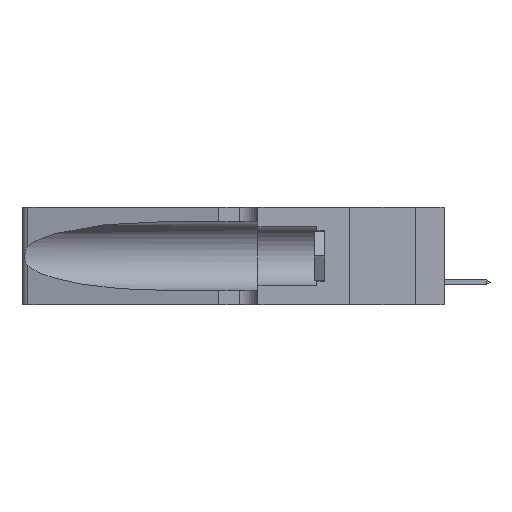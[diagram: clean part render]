
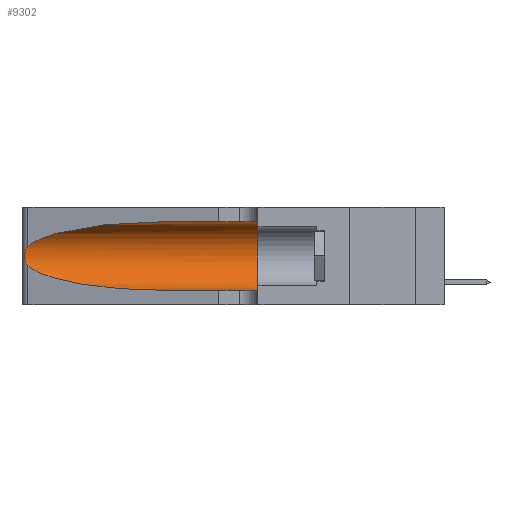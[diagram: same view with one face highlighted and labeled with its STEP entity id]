
A CAD part, left-side view. The second image highlights one B-rep face of the part: STEP entity #9302.
In plain terms, the highlighted cylindrical face has radius 3.308 mm (diameter 6.617 mm), a partial arc.
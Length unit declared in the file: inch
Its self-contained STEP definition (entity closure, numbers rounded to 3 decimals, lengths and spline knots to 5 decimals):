
#2052 = CARTESIAN_POINT ( 'NONE',  ( 0.26075, 1.23896, 0.19203 ) ) ;
#2098 = CARTESIAN_POINT ( 'NONE',  ( 0.2373, 1.15595, 0.08982 ) ) ;
#3570 = CARTESIAN_POINT ( 'NONE',  ( 0.25487, 1.22718, 0.14631 ) ) ;
#4041 = CARTESIAN_POINT ( 'NONE',  ( 0.1305, 0.35, 0.185 ) ) ;
#4953 = CARTESIAN_POINT ( 'NONE',  ( 0.26017, 1.23833, 0.17102 ) ) ;
#5603 = VERTEX_POINT ( 'NONE', #26586 ) ;
#6183 = VERTEX_POINT ( 'NONE', #3570 ) ;
#6469 = CARTESIAN_POINT ( 'NONE',  ( 0.1305, 0.35, 0.31525 ) ) ;
#6683 = VERTEX_POINT ( 'NONE', #33255 ) ;
#7606 = EDGE_CURVE ( 'NONE', #20754, #26557, #24530, .T. ) ;
#7686 = CARTESIAN_POINT ( 'NONE',  ( 0.18966, 0.96281, 0.05475 ) ) ;
#7894 = CARTESIAN_POINT ( 'NONE',  ( 0.25639, 1.23184, 0.21858 ) ) ;
#8058 = CARTESIAN_POINT ( 'NONE',  ( 0.25487, 1.22718, 0.14631 ) ) ;
#9302 = ADVANCED_FACE ( 'NONE', ( #12553 ), #36191, .F. ) ;
#10468 = CARTESIAN_POINT ( 'NONE',  ( 0.25787, 1.23484, 0.2124 ) ) ;
#10715 = CARTESIAN_POINT ( 'NONE',  ( 0.25854, 1.2359, 0.20912 ) ) ;
#10852 = CARTESIAN_POINT ( 'NONE',  ( 0.25856, 1.23593, 0.16098 ) ) ;
#10862 = AXIS2_PLACEMENT_3D ( 'NONE', #4041, #15674, #12991 ) ;
#11027 = CARTESIAN_POINT ( 'NONE',  ( 0.1305, 0.72297, 0.05475 ) ) ;
#11537 = B_SPLINE_CURVE_WITH_KNOTS ( 'NONE', 3,
 ( #13523, #28240, #7894, #10468, #10715, #31073, #2052, #22396, #4953, #10852, #16465, #13778, #33866, #22278 ),
 .UNSPECIFIED., .F., .F.,
 ( 4, 2, 2, 2, 2, 2, 4 ),
 ( 0., 0.00027, 0.00053, 0.00107, 0.0016, 0.00187, 0.00214 ),
 .UNSPECIFIED. ) ;
#11784 = CARTESIAN_POINT ( 'NONE',  ( 0.25487, 1.22718, 0.22369 ) ) ;
#12470 = VECTOR ( 'NONE', #30517, 39.37008 ) ;
#12553 = FACE_OUTER_BOUND ( 'NONE', #32951, .T. ) ;
#12991 = DIRECTION ( 'NONE',  ( 0., 0., 1. ) ) ;
#13214 = CARTESIAN_POINT ( 'NONE',  ( 0.1305, 0.72297, 0.31525 ) ) ;
#13523 = CARTESIAN_POINT ( 'NONE',  ( 0.25487, 1.22718, 0.22369 ) ) ;
#13662 = CARTESIAN_POINT ( 'NONE',  ( 0.1305, 1.61858, 0.185 ) ) ;
#13778 = CARTESIAN_POINT ( 'NONE',  ( 0.25639, 1.23186, 0.15144 ) ) ;
#13784 = VECTOR ( 'NONE', #30299, 39.37008 ) ;
#15674 = DIRECTION ( 'NONE',  ( 0., 1., 0. ) ) ;
#16164 = EDGE_CURVE ( 'NONE', #26557, #6183, #11537, .T. ) ;
#16174 = AXIS2_PLACEMENT_3D ( 'NONE', #13662, #37060, #19612 ) ;
#16465 = CARTESIAN_POINT ( 'NONE',  ( 0.25789, 1.23486, 0.15765 ) ) ;
#16741 = ORIENTED_EDGE ( 'NONE', *, *, #19785, .F. ) ;
#17801 =( BOUNDED_CURVE ( )  B_SPLINE_CURVE ( 3, ( #8058, #2098, #7686, #11027 ),
 .UNSPECIFIED., .F., .F. ) 
 B_SPLINE_CURVE_WITH_KNOTS ( ( 4, 4 ),
 ( 3.44316, 4.71239 ),
 .UNSPECIFIED. ) 
 CURVE ( )  GEOMETRIC_REPRESENTATION_ITEM ( )  RATIONAL_B_SPLINE_CURVE ( ( 1., 0.87, 0.87, 1. ) ) 
 REPRESENTATION_ITEM ( '' )  );
#18469 = CARTESIAN_POINT ( 'NONE',  ( 0.18966, 0.96281, 0.31525 ) ) ;
#18583 = CARTESIAN_POINT ( 'NONE',  ( 0.2373, 1.15595, 0.28018 ) ) ;
#18840 = CARTESIAN_POINT ( 'NONE',  ( 0.25487, 1.22718, 0.22369 ) ) ;
#19612 = DIRECTION ( 'NONE',  ( 0., 0., -1. ) ) ;
#19785 = EDGE_CURVE ( 'NONE', #20754, #27251, #35129, .T. ) ;
#20754 = VERTEX_POINT ( 'NONE', #13214 ) ;
#22278 = CARTESIAN_POINT ( 'NONE',  ( 0.25487, 1.22718, 0.14631 ) ) ;
#22396 = CARTESIAN_POINT ( 'NONE',  ( 0.26075, 1.23896, 0.178 ) ) ;
#22849 = EDGE_CURVE ( 'NONE', #6183, #6683, #17801, .T. ) ;
#23827 = EDGE_CURVE ( 'NONE', #6683, #5603, #36107, .T. ) ;
#24530 =( BOUNDED_CURVE ( )  B_SPLINE_CURVE ( 3, ( #27475, #18469, #18583, #18840 ),
 .UNSPECIFIED., .F., .F. ) 
 B_SPLINE_CURVE_WITH_KNOTS ( ( 4, 4 ),
 ( 1.5708, 2.84003 ),
 .UNSPECIFIED. ) 
 CURVE ( )  GEOMETRIC_REPRESENTATION_ITEM ( )  RATIONAL_B_SPLINE_CURVE ( ( 1., 0.87, 0.87, 1. ) ) 
 REPRESENTATION_ITEM ( '' )  );
#26557 = VERTEX_POINT ( 'NONE', #11784 ) ;
#26586 = CARTESIAN_POINT ( 'NONE',  ( 0.1305, 0.35, 0.05475 ) ) ;
#27251 = VERTEX_POINT ( 'NONE', #6469 ) ;
#27475 = CARTESIAN_POINT ( 'NONE',  ( 0.1305, 0.72297, 0.31525 ) ) ;
#28240 = CARTESIAN_POINT ( 'NONE',  ( 0.25555, 1.22994, 0.2215 ) ) ;
#28391 = ORIENTED_EDGE ( 'NONE', *, *, #22849, .T. ) ;
#28420 = ORIENTED_EDGE ( 'NONE', *, *, #16164, .T. ) ;
#30299 = DIRECTION ( 'NONE',  ( 0., -1., 0. ) ) ;
#30517 = DIRECTION ( 'NONE',  ( 0., -1., 0. ) ) ;
#31073 = CARTESIAN_POINT ( 'NONE',  ( 0.26018, 1.23835, 0.19895 ) ) ;
#32101 = EDGE_CURVE ( 'NONE', #27251, #5603, #33586, .T. ) ;
#32935 = CARTESIAN_POINT ( 'NONE',  ( 0.1305, 1.61858, 0.05475 ) ) ;
#32951 = EDGE_LOOP ( 'NONE', ( #35219, #28420, #28391, #34646, #33356, #16741 ) ) ;
#33096 = CARTESIAN_POINT ( 'NONE',  ( 0.1305, 1.61858, 0.31525 ) ) ;
#33255 = CARTESIAN_POINT ( 'NONE',  ( 0.1305, 0.72297, 0.05475 ) ) ;
#33356 = ORIENTED_EDGE ( 'NONE', *, *, #32101, .F. ) ;
#33586 = CIRCLE ( 'NONE', #10862, 0.13025 ) ;
#33866 = CARTESIAN_POINT ( 'NONE',  ( 0.25555, 1.22993, 0.14849 ) ) ;
#34646 = ORIENTED_EDGE ( 'NONE', *, *, #23827, .T. ) ;
#35129 = LINE ( 'NONE', #33096, #13784 ) ;
#35219 = ORIENTED_EDGE ( 'NONE', *, *, #7606, .T. ) ;
#36107 = LINE ( 'NONE', #32935, #12470 ) ;
#36191 = CYLINDRICAL_SURFACE ( 'NONE', #16174, 0.13025 ) ;
#37060 = DIRECTION ( 'NONE',  ( 0., -1., 0. ) ) ;
